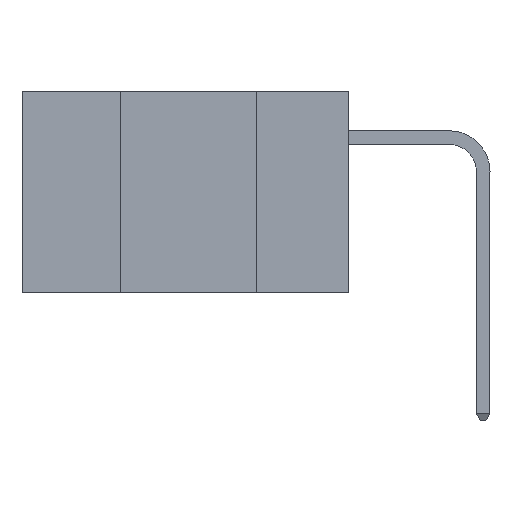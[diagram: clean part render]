
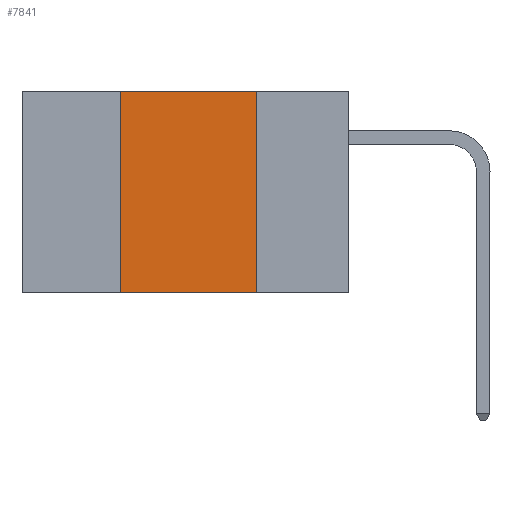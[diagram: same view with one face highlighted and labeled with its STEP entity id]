
A CAD part, left-side view. The second image highlights one B-rep face of the part: STEP entity #7841.
In plain terms, the highlighted planar face has unit normal (-1, 0, 0).
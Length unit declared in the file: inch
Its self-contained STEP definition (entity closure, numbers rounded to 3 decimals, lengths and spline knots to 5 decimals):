
#1086 = DIRECTION ( 'NONE',  ( 0., 0., -1. ) ) ;
#3510 = CARTESIAN_POINT ( 'NONE',  ( 0., 0.42, -0.37 ) ) ;
#4512 = ORIENTED_EDGE ( 'NONE', *, *, #27803, .F. ) ;
#7753 = VERTEX_POINT ( 'NONE', #23379 ) ;
#7841 = ADVANCED_FACE ( 'NONE', ( #15403 ), #15229, .F. ) ;
#8716 = CARTESIAN_POINT ( 'NONE',  ( 0., 0.17, 0. ) ) ;
#9347 = VECTOR ( 'NONE', #28394, 39.37008 ) ;
#11982 = VERTEX_POINT ( 'NONE', #3510 ) ;
#12777 = VECTOR ( 'NONE', #27400, 39.37008 ) ;
#15229 = PLANE ( 'NONE',  #32889 ) ;
#15403 = FACE_OUTER_BOUND ( 'NONE', #25777, .T. ) ;
#16012 = CARTESIAN_POINT ( 'NONE',  ( 0., 0.42, 0. ) ) ;
#17579 = LINE ( 'NONE', #16012, #31437 ) ;
#17665 = LINE ( 'NONE', #31169, #9347 ) ;
#18164 = DIRECTION ( 'NONE',  ( 1., 0., 0. ) ) ;
#18798 = DIRECTION ( 'NONE',  ( 0., 0., 1. ) ) ;
#18953 = LINE ( 'NONE', #23655, #31087 ) ;
#21635 = EDGE_CURVE ( 'NONE', #7753, #34959, #27575, .T. ) ;
#23379 = CARTESIAN_POINT ( 'NONE',  ( 0., 0.42, 0. ) ) ;
#23426 = CARTESIAN_POINT ( 'NONE',  ( 0., 0.17, -0.37 ) ) ;
#23527 = ORIENTED_EDGE ( 'NONE', *, *, #32257, .F. ) ;
#23655 = CARTESIAN_POINT ( 'NONE',  ( 0., 0.6, -0.37 ) ) ;
#25777 = EDGE_LOOP ( 'NONE', ( #23527, #33473, #4512, #26828 ) ) ;
#26828 = ORIENTED_EDGE ( 'NONE', *, *, #32460, .T. ) ;
#27400 = DIRECTION ( 'NONE',  ( 0., -1., 0. ) ) ;
#27575 = LINE ( 'NONE', #30294, #12777 ) ;
#27803 = EDGE_CURVE ( 'NONE', #11982, #7753, #17579, .T. ) ;
#28394 = DIRECTION ( 'NONE',  ( 0., 0., -1. ) ) ;
#30294 = CARTESIAN_POINT ( 'NONE',  ( 0., 0.6, 0. ) ) ;
#31087 = VECTOR ( 'NONE', #31981, 39.37008 ) ;
#31169 = CARTESIAN_POINT ( 'NONE',  ( 0., 0.17, 0. ) ) ;
#31437 = VECTOR ( 'NONE', #18798, 39.37008 ) ;
#31981 = DIRECTION ( 'NONE',  ( 0., -1., 0. ) ) ;
#32257 = EDGE_CURVE ( 'NONE', #34959, #34341, #17665, .T. ) ;
#32460 = EDGE_CURVE ( 'NONE', #11982, #34341, #18953, .T. ) ;
#32889 = AXIS2_PLACEMENT_3D ( 'NONE', #34657, #18164, #1086 ) ;
#33473 = ORIENTED_EDGE ( 'NONE', *, *, #21635, .F. ) ;
#34341 = VERTEX_POINT ( 'NONE', #23426 ) ;
#34657 = CARTESIAN_POINT ( 'NONE',  ( 0., 0.6, 0. ) ) ;
#34959 = VERTEX_POINT ( 'NONE', #8716 ) ;
